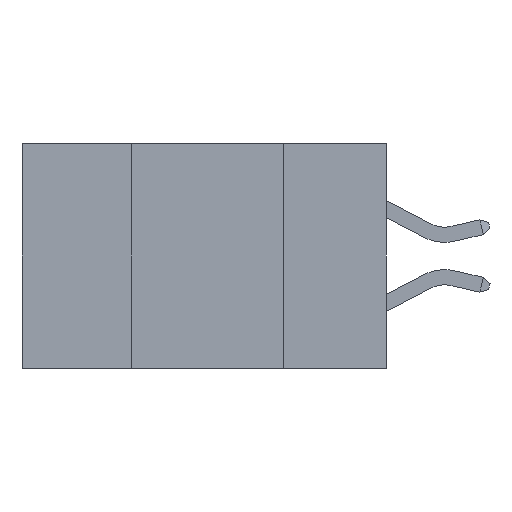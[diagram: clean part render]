
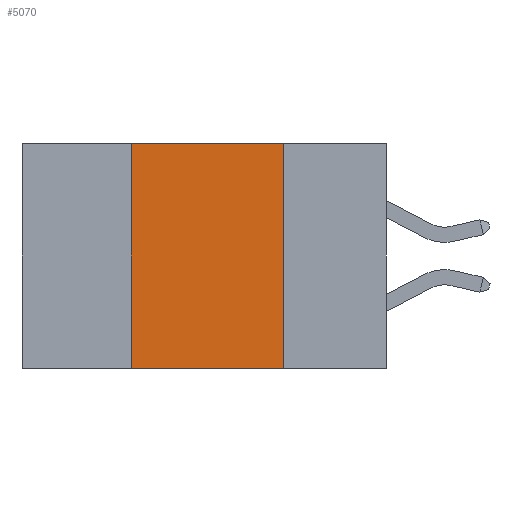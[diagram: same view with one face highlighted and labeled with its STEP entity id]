
A CAD part, left-side view. The second image highlights one B-rep face of the part: STEP entity #5070.
In plain terms, the highlighted planar face has unit normal (-1, 0, 0).
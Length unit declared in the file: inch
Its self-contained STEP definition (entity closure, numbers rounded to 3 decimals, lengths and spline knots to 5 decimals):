
#85 = VECTOR ( 'NONE', #7090, 39.37008 ) ;
#88 = ORIENTED_EDGE ( 'NONE', *, *, #4259, .F. ) ;
#541 = EDGE_CURVE ( 'NONE', #14190, #4902, #661, .T. ) ;
#661 = LINE ( 'NONE', #683, #4332 ) ;
#683 = CARTESIAN_POINT ( 'NONE',  ( 0., 0.6, -0.37 ) ) ;
#816 = EDGE_CURVE ( 'NONE', #3595, #8134, #854, .T. ) ;
#846 = VECTOR ( 'NONE', #6318, 39.37008 ) ;
#851 = CARTESIAN_POINT ( 'NONE',  ( 0., 0.17, -0.37 ) ) ;
#854 = LINE ( 'NONE', #866, #85 ) ;
#866 = CARTESIAN_POINT ( 'NONE',  ( 0., 0.6, 0. ) ) ;
#880 = DIRECTION ( 'NONE',  ( 0., 0., -1. ) ) ;
#898 = DIRECTION ( 'NONE',  ( 0., 0., -1. ) ) ;
#915 = DIRECTION ( 'NONE',  ( 1., 0., 0. ) ) ;
#1256 = CARTESIAN_POINT ( 'NONE',  ( 0., 0.6, 0. ) ) ;
#1295 = LINE ( 'NONE', #851, #4212 ) ;
#1668 = AXIS2_PLACEMENT_3D ( 'NONE', #1256, #915, #898 ) ;
#2371 = PLANE ( 'NONE',  #1668 ) ;
#3353 = ORIENTED_EDGE ( 'NONE', *, *, #816, .F. ) ;
#3595 = VERTEX_POINT ( 'NONE', #6315 ) ;
#4212 = VECTOR ( 'NONE', #880, 39.37008 ) ;
#4259 = EDGE_CURVE ( 'NONE', #8134, #4902, #1295, .T. ) ;
#4332 = VECTOR ( 'NONE', #5532, 39.37008 ) ;
#4902 = VERTEX_POINT ( 'NONE', #7318 ) ;
#5070 = ADVANCED_FACE ( 'NONE', ( #11980 ), #2371, .F. ) ;
#5112 = CARTESIAN_POINT ( 'NONE',  ( 0., 0.42, -0.37 ) ) ;
#5532 = DIRECTION ( 'NONE',  ( 0., -1., 0. ) ) ;
#5818 = EDGE_LOOP ( 'NONE', ( #88, #3353, #9803, #12806 ) ) ;
#6315 = CARTESIAN_POINT ( 'NONE',  ( 0., 0.42, 0. ) ) ;
#6318 = DIRECTION ( 'NONE',  ( 0., 0., 1. ) ) ;
#6663 = CARTESIAN_POINT ( 'NONE',  ( 0., 0.42, -0.37 ) ) ;
#7090 = DIRECTION ( 'NONE',  ( 0., -1., 0. ) ) ;
#7135 = CARTESIAN_POINT ( 'NONE',  ( 0., 0.17, 0. ) ) ;
#7318 = CARTESIAN_POINT ( 'NONE',  ( 0., 0.17, -0.37 ) ) ;
#7341 = LINE ( 'NONE', #5112, #846 ) ;
#8134 = VERTEX_POINT ( 'NONE', #7135 ) ;
#9803 = ORIENTED_EDGE ( 'NONE', *, *, #13040, .F. ) ;
#11980 = FACE_OUTER_BOUND ( 'NONE', #5818, .T. ) ;
#12806 = ORIENTED_EDGE ( 'NONE', *, *, #541, .T. ) ;
#13040 = EDGE_CURVE ( 'NONE', #14190, #3595, #7341, .T. ) ;
#14190 = VERTEX_POINT ( 'NONE', #6663 ) ;
